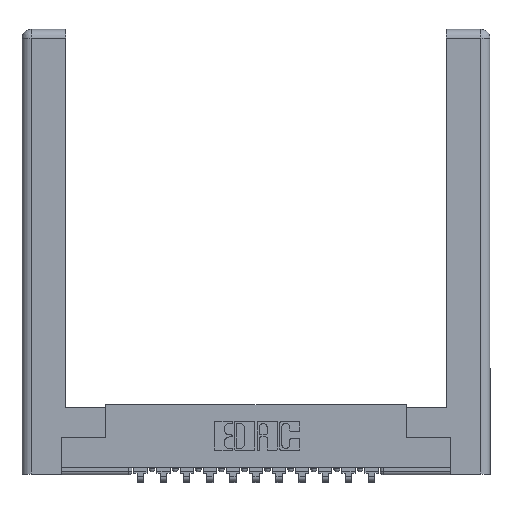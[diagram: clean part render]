
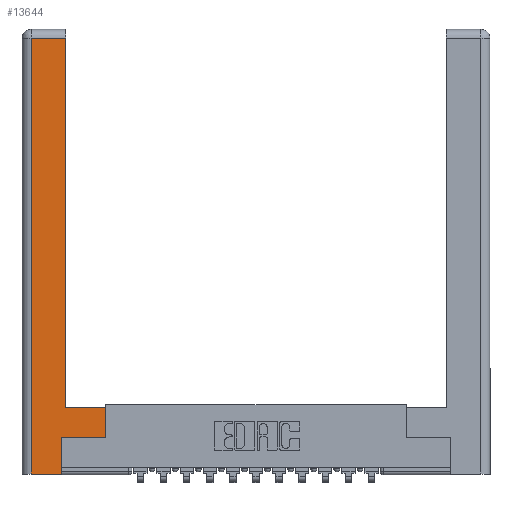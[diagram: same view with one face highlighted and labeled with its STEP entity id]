
A CAD part, top view. The second image highlights one B-rep face of the part: STEP entity #13644.
In plain terms, the highlighted planar face has unit normal (0, 0, 1).
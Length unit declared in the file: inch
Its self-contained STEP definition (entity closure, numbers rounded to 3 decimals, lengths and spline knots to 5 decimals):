
#78 = LINE ( 'NONE', #2488, #12975 ) ;
#450 = ORIENTED_EDGE ( 'NONE', *, *, #5585, .T. ) ;
#657 = CARTESIAN_POINT ( 'NONE',  ( 0.265, 0.245, 0. ) ) ;
#830 = ORIENTED_EDGE ( 'NONE', *, *, #6026, .T. ) ;
#887 = ORIENTED_EDGE ( 'NONE', *, *, #4744, .T. ) ;
#904 = VERTEX_POINT ( 'NONE', #3299 ) ;
#2488 = CARTESIAN_POINT ( 'NONE',  ( 0.265, 0.245, 0. ) ) ;
#2504 = CARTESIAN_POINT ( 'NONE',  ( 0.295, 0.45, 0. ) ) ;
#2716 = EDGE_CURVE ( 'NONE', #2999, #16400, #4553, .T. ) ;
#2824 = VERTEX_POINT ( 'NONE', #2504 ) ;
#2999 = VERTEX_POINT ( 'NONE', #8271 ) ;
#3236 = CARTESIAN_POINT ( 'NONE',  ( 0.295, 3., 0. ) ) ;
#3275 = ORIENTED_EDGE ( 'NONE', *, *, #8596, .T. ) ;
#3299 = CARTESIAN_POINT ( 'NONE',  ( 0.265, 0., 0. ) ) ;
#3422 = CARTESIAN_POINT ( 'NONE',  ( 0., 0., 0. ) ) ;
#3467 = DIRECTION ( 'NONE',  ( 0., 1., 0. ) ) ;
#3808 = VERTEX_POINT ( 'NONE', #11621 ) ;
#4282 = VECTOR ( 'NONE', #16297, 39.37008 ) ;
#4553 = LINE ( 'NONE', #4639, #5367 ) ;
#4599 = EDGE_CURVE ( 'NONE', #13777, #3808, #16255, .T. ) ;
#4605 = PLANE ( 'NONE',  #4988 ) ;
#4617 = ORIENTED_EDGE ( 'NONE', *, *, #4623, .T. ) ;
#4623 = EDGE_CURVE ( 'NONE', #3808, #2824, #11171, .T. ) ;
#4639 = CARTESIAN_POINT ( 'NONE',  ( 0.0615, 2.94, 0. ) ) ;
#4744 = EDGE_CURVE ( 'NONE', #904, #6633, #78, .T. ) ;
#4988 = AXIS2_PLACEMENT_3D ( 'NONE', #3422, #12411, #13730 ) ;
#5367 = VECTOR ( 'NONE', #15119, 39.37008 ) ;
#5585 = EDGE_CURVE ( 'NONE', #2824, #2999, #16034, .T. ) ;
#5762 = CARTESIAN_POINT ( 'NONE',  ( 0.0615, 2.94, 0. ) ) ;
#5981 = EDGE_CURVE ( 'NONE', #16400, #14119, #12714, .T. ) ;
#6014 = CARTESIAN_POINT ( 'NONE',  ( 0.265, 0., 0. ) ) ;
#6026 = EDGE_CURVE ( 'NONE', #6633, #13777, #7060, .T. ) ;
#6428 = ORIENTED_EDGE ( 'NONE', *, *, #4599, .T. ) ;
#6501 = VECTOR ( 'NONE', #10524, 39.37008 ) ;
#6633 = VERTEX_POINT ( 'NONE', #657 ) ;
#7060 = LINE ( 'NONE', #14529, #9687 ) ;
#7113 = VECTOR ( 'NONE', #3467, 39.37008 ) ;
#7783 = CARTESIAN_POINT ( 'NONE',  ( 0.565, 0.245, 0. ) ) ;
#7857 = VECTOR ( 'NONE', #8275, 39.37008 ) ;
#8271 = CARTESIAN_POINT ( 'NONE',  ( 0.295, 2.94, 0. ) ) ;
#8275 = DIRECTION ( 'NONE',  ( 0., -1., 0. ) ) ;
#8596 = EDGE_CURVE ( 'NONE', #14119, #904, #11387, .T. ) ;
#8795 = CARTESIAN_POINT ( 'NONE',  ( 0.295, 0.45, 0. ) ) ;
#8891 = VECTOR ( 'NONE', #12391, 39.37008 ) ;
#9008 = DIRECTION ( 'NONE',  ( 0., 1., 0. ) ) ;
#9687 = VECTOR ( 'NONE', #12197, 39.37008 ) ;
#10524 = DIRECTION ( 'NONE',  ( -1., 0., 0. ) ) ;
#11171 = LINE ( 'NONE', #8795, #6501 ) ;
#11387 = LINE ( 'NONE', #6014, #4282 ) ;
#11597 = ORIENTED_EDGE ( 'NONE', *, *, #2716, .T. ) ;
#11621 = CARTESIAN_POINT ( 'NONE',  ( 0.565, 0.45, 0. ) ) ;
#11899 = ORIENTED_EDGE ( 'NONE', *, *, #5981, .T. ) ;
#12108 = FACE_OUTER_BOUND ( 'NONE', #14637, .T. ) ;
#12197 = DIRECTION ( 'NONE',  ( 1., 0., 0. ) ) ;
#12391 = DIRECTION ( 'NONE',  ( 0., 1., 0. ) ) ;
#12411 = DIRECTION ( 'NONE',  ( 0., 0., -1. ) ) ;
#12714 = LINE ( 'NONE', #14582, #7857 ) ;
#12975 = VECTOR ( 'NONE', #9008, 39.37008 ) ;
#13644 = ADVANCED_FACE ( 'NONE', ( #12108 ), #4605, .F. ) ;
#13730 = DIRECTION ( 'NONE',  ( -1., 0., 0. ) ) ;
#13766 = CARTESIAN_POINT ( 'NONE',  ( 0.565, 0.45, 0. ) ) ;
#13777 = VERTEX_POINT ( 'NONE', #7783 ) ;
#14119 = VERTEX_POINT ( 'NONE', #16393 ) ;
#14529 = CARTESIAN_POINT ( 'NONE',  ( 0.565, 0.245, 0. ) ) ;
#14582 = CARTESIAN_POINT ( 'NONE',  ( 0.0615, 0., 0. ) ) ;
#14637 = EDGE_LOOP ( 'NONE', ( #450, #11597, #11899, #3275, #887, #830, #6428, #4617 ) ) ;
#15119 = DIRECTION ( 'NONE',  ( -1., 0., 0. ) ) ;
#16034 = LINE ( 'NONE', #3236, #8891 ) ;
#16255 = LINE ( 'NONE', #13766, #7113 ) ;
#16297 = DIRECTION ( 'NONE',  ( 1., 0., 0. ) ) ;
#16393 = CARTESIAN_POINT ( 'NONE',  ( 0.0615, 0., 0. ) ) ;
#16400 = VERTEX_POINT ( 'NONE', #5762 ) ;
